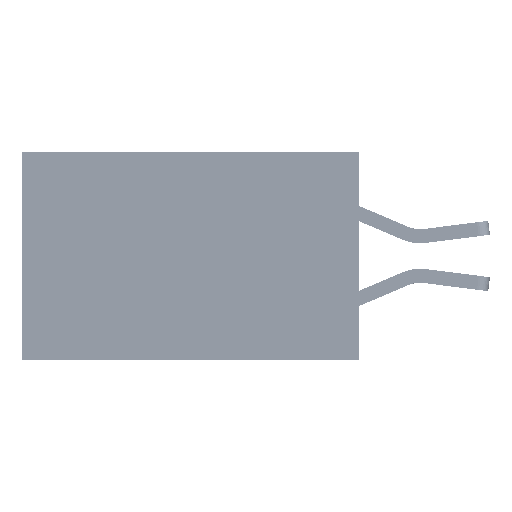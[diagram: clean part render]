
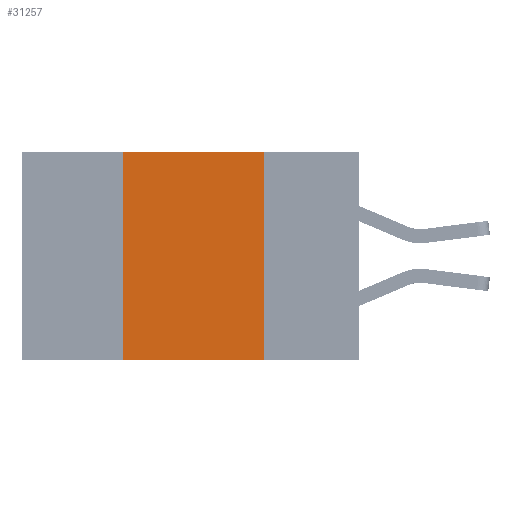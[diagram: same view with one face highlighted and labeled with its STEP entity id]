
A CAD part, left-side view. The second image highlights one B-rep face of the part: STEP entity #31257.
In plain terms, the highlighted planar face has unit normal (-1, 0, 0).
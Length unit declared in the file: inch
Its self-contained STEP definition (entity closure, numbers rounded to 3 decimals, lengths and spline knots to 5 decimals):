
#126 = ORIENTED_EDGE ( 'NONE', *, *, #25998, .T. ) ;
#503 = CARTESIAN_POINT ( 'NONE',  ( 0., 0.17, 0. ) ) ;
#3138 = CARTESIAN_POINT ( 'NONE',  ( 0., 0.42, -0.37 ) ) ;
#3353 = DIRECTION ( 'NONE',  ( 1., 0., 0. ) ) ;
#4411 = ORIENTED_EDGE ( 'NONE', *, *, #30907, .F. ) ;
#4914 = CARTESIAN_POINT ( 'NONE',  ( 0., 0.17, -0.37 ) ) ;
#5895 = ORIENTED_EDGE ( 'NONE', *, *, #8924, .F. ) ;
#5959 = DIRECTION ( 'NONE',  ( 0., -1., 0. ) ) ;
#7398 = VECTOR ( 'NONE', #9138, 39.37008 ) ;
#7550 = VECTOR ( 'NONE', #20098, 39.37008 ) ;
#7842 = CARTESIAN_POINT ( 'NONE',  ( 0., 0.42, 0. ) ) ;
#8924 = EDGE_CURVE ( 'NONE', #17394, #32639, #30739, .T. ) ;
#9138 = DIRECTION ( 'NONE',  ( 0., -1., 0. ) ) ;
#9441 = VECTOR ( 'NONE', #26641, 39.37008 ) ;
#10715 = ORIENTED_EDGE ( 'NONE', *, *, #24052, .F. ) ;
#12397 = EDGE_LOOP ( 'NONE', ( #10715, #4411, #5895, #126 ) ) ;
#14910 = DIRECTION ( 'NONE',  ( 0., 0., -1. ) ) ;
#17394 = VERTEX_POINT ( 'NONE', #3138 ) ;
#19010 = AXIS2_PLACEMENT_3D ( 'NONE', #37195, #3353, #14910 ) ;
#20098 = DIRECTION ( 'NONE',  ( 0., 0., -1. ) ) ;
#24025 = LINE ( 'NONE', #39704, #45341 ) ;
#24052 = EDGE_CURVE ( 'NONE', #30253, #34890, #34170, .T. ) ;
#24700 = CARTESIAN_POINT ( 'NONE',  ( 0., 0.6, 0. ) ) ;
#25998 = EDGE_CURVE ( 'NONE', #17394, #34890, #24025, .T. ) ;
#26641 = DIRECTION ( 'NONE',  ( 0., 0., 1. ) ) ;
#29284 = LINE ( 'NONE', #24700, #7398 ) ;
#30253 = VERTEX_POINT ( 'NONE', #503 ) ;
#30739 = LINE ( 'NONE', #41870, #9441 ) ;
#30907 = EDGE_CURVE ( 'NONE', #32639, #30253, #29284, .T. ) ;
#31257 = ADVANCED_FACE ( 'NONE', ( #47646 ), #33239, .F. ) ;
#32639 = VERTEX_POINT ( 'NONE', #7842 ) ;
#33239 = PLANE ( 'NONE',  #19010 ) ;
#34170 = LINE ( 'NONE', #46928, #7550 ) ;
#34890 = VERTEX_POINT ( 'NONE', #4914 ) ;
#37195 = CARTESIAN_POINT ( 'NONE',  ( 0., 0.6, 0. ) ) ;
#39704 = CARTESIAN_POINT ( 'NONE',  ( 0., 0.6, -0.37 ) ) ;
#41870 = CARTESIAN_POINT ( 'NONE',  ( 0., 0.42, 0. ) ) ;
#45341 = VECTOR ( 'NONE', #5959, 39.37008 ) ;
#46928 = CARTESIAN_POINT ( 'NONE',  ( 0., 0.17, 0. ) ) ;
#47646 = FACE_OUTER_BOUND ( 'NONE', #12397, .T. ) ;
